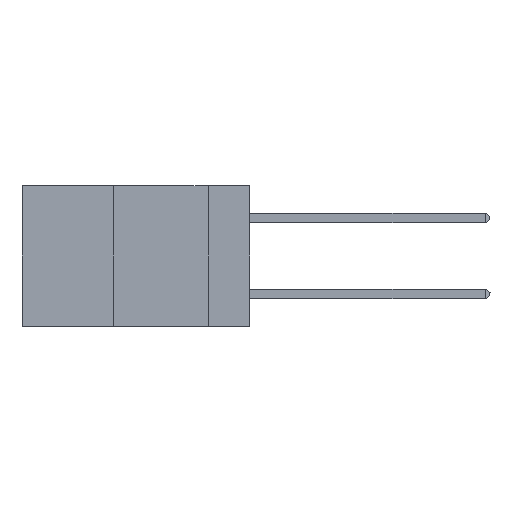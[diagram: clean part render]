
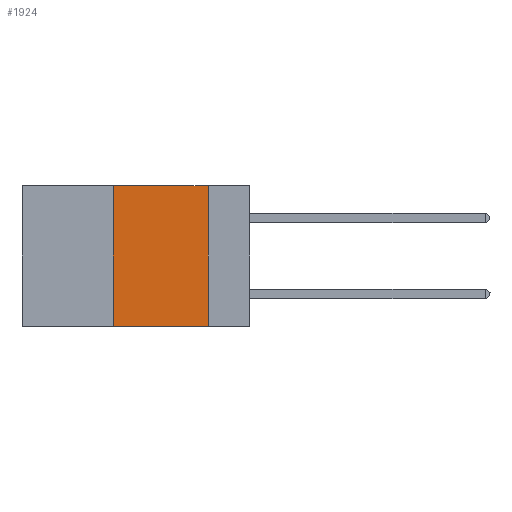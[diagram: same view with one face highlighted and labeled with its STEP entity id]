
A CAD part, left-side view. The second image highlights one B-rep face of the part: STEP entity #1924.
In plain terms, the highlighted planar face has unit normal (-1, 0, 0).
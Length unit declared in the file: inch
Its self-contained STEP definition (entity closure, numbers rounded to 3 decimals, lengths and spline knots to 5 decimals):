
#178 = VERTEX_POINT ( 'NONE', #8175 ) ;
#475 = LINE ( 'NONE', #19901, #16768 ) ;
#876 = EDGE_CURVE ( 'NONE', #26503, #178, #475, .T. ) ;
#1924 = ADVANCED_FACE ( 'NONE', ( #19583 ), #5622, .F. ) ;
#2608 = ORIENTED_EDGE ( 'NONE', *, *, #3995, .F. ) ;
#3558 = EDGE_LOOP ( 'NONE', ( #3817, #8671, #2608, #25482 ) ) ;
#3817 = ORIENTED_EDGE ( 'NONE', *, *, #876, .F. ) ;
#3995 = EDGE_CURVE ( 'NONE', #21389, #20310, #6109, .T. ) ;
#5622 = PLANE ( 'NONE',  #23564 ) ;
#6109 = LINE ( 'NONE', #26340, #9821 ) ;
#7784 = DIRECTION ( 'NONE',  ( 1., 0., 0. ) ) ;
#8144 = VECTOR ( 'NONE', #14153, 39.37008 ) ;
#8175 = CARTESIAN_POINT ( 'NONE',  ( 0., 0.11, -0.37 ) ) ;
#8671 = ORIENTED_EDGE ( 'NONE', *, *, #22382, .F. ) ;
#9821 = VECTOR ( 'NONE', #20260, 39.37008 ) ;
#9875 = LINE ( 'NONE', #24012, #24367 ) ;
#10907 = CARTESIAN_POINT ( 'NONE',  ( 0., 0.11, 0. ) ) ;
#13058 = CARTESIAN_POINT ( 'NONE',  ( 0., 0.36, 0. ) ) ;
#14153 = DIRECTION ( 'NONE',  ( 0., -1., 0. ) ) ;
#16768 = VECTOR ( 'NONE', #25136, 39.37008 ) ;
#18978 = EDGE_CURVE ( 'NONE', #21389, #178, #19851, .T. ) ;
#19583 = FACE_OUTER_BOUND ( 'NONE', #3558, .T. ) ;
#19851 = LINE ( 'NONE', #24331, #8144 ) ;
#19901 = CARTESIAN_POINT ( 'NONE',  ( 0., 0.11, 0. ) ) ;
#20260 = DIRECTION ( 'NONE',  ( 0., 0., 1. ) ) ;
#20269 = CARTESIAN_POINT ( 'NONE',  ( 0., 0.6, 0. ) ) ;
#20310 = VERTEX_POINT ( 'NONE', #13058 ) ;
#21389 = VERTEX_POINT ( 'NONE', #26966 ) ;
#22310 = DIRECTION ( 'NONE',  ( 0., 0., -1. ) ) ;
#22382 = EDGE_CURVE ( 'NONE', #20310, #26503, #9875, .T. ) ;
#23564 = AXIS2_PLACEMENT_3D ( 'NONE', #20269, #7784, #22310 ) ;
#24012 = CARTESIAN_POINT ( 'NONE',  ( 0., 0.6, 0. ) ) ;
#24331 = CARTESIAN_POINT ( 'NONE',  ( 0., 0.6, -0.37 ) ) ;
#24367 = VECTOR ( 'NONE', #26091, 39.37008 ) ;
#25136 = DIRECTION ( 'NONE',  ( 0., 0., -1. ) ) ;
#25482 = ORIENTED_EDGE ( 'NONE', *, *, #18978, .T. ) ;
#26091 = DIRECTION ( 'NONE',  ( 0., -1., 0. ) ) ;
#26340 = CARTESIAN_POINT ( 'NONE',  ( 0., 0.36, 0. ) ) ;
#26503 = VERTEX_POINT ( 'NONE', #10907 ) ;
#26966 = CARTESIAN_POINT ( 'NONE',  ( 0., 0.36, -0.37 ) ) ;
